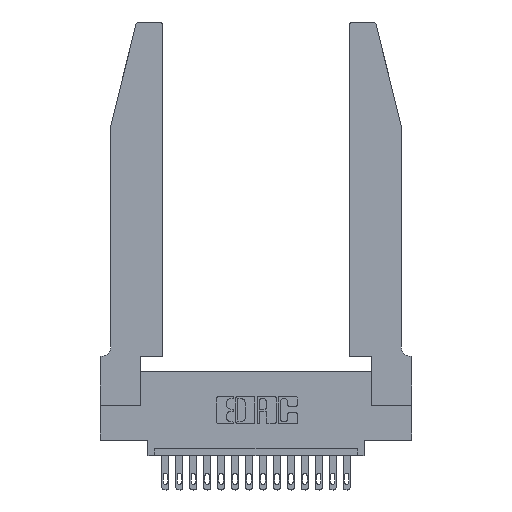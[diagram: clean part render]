
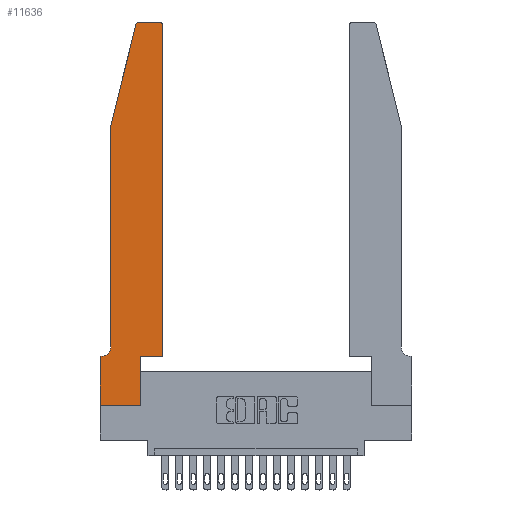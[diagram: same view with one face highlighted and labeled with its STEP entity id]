
A CAD part, top view. The second image highlights one B-rep face of the part: STEP entity #11636.
In plain terms, the highlighted planar face has unit normal (0, 0, 1).
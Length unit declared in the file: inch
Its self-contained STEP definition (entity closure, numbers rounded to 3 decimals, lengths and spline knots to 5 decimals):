
#228 = DIRECTION ( 'NONE',  ( 0., 0., 1. ) ) ;
#827 = LINE ( 'NONE', #8699, #14005 ) ;
#877 = DIRECTION ( 'NONE',  ( 1., 0., 0. ) ) ;
#1120 = VERTEX_POINT ( 'NONE', #11912 ) ;
#1495 = ORIENTED_EDGE ( 'NONE', *, *, #17702, .T. ) ;
#1582 = EDGE_CURVE ( 'NONE', #5676, #4502, #16400, .T. ) ;
#1652 = ORIENTED_EDGE ( 'NONE', *, *, #2172, .T. ) ;
#1903 = VECTOR ( 'NONE', #17147, 39.37008 ) ;
#2052 = VECTOR ( 'NONE', #2347, 39.37008 ) ;
#2172 = EDGE_CURVE ( 'NONE', #15563, #7619, #3936, .T. ) ;
#2191 = EDGE_CURVE ( 'NONE', #11551, #15723, #13420, .T. ) ;
#2324 = VERTEX_POINT ( 'NONE', #4668 ) ;
#2347 = DIRECTION ( 'NONE',  ( -1., 0., 0. ) ) ;
#2508 = EDGE_CURVE ( 'NONE', #11170, #12151, #18224, .T. ) ;
#2566 = VERTEX_POINT ( 'NONE', #10571 ) ;
#2776 = DIRECTION ( 'NONE',  ( 0., 1., 0. ) ) ;
#2810 = VERTEX_POINT ( 'NONE', #17596 ) ;
#2913 = LINE ( 'NONE', #4439, #18145 ) ;
#3308 = LINE ( 'NONE', #15103, #14832 ) ;
#3457 = DIRECTION ( 'NONE',  ( -1., 0., 0. ) ) ;
#3936 = CIRCLE ( 'NONE', #7924, 0.03 ) ;
#4192 = CARTESIAN_POINT ( 'NONE',  ( 0.4505, 0.35, 0.37 ) ) ;
#4439 = CARTESIAN_POINT ( 'NONE',  ( 0.2865, 0.35, 0.37 ) ) ;
#4440 = EDGE_CURVE ( 'NONE', #1120, #2810, #827, .T. ) ;
#4502 = VERTEX_POINT ( 'NONE', #7293 ) ;
#4646 = CARTESIAN_POINT ( 'NONE',  ( 0.4205, 2.75, 0.37 ) ) ;
#4668 = CARTESIAN_POINT ( 'NONE',  ( 0.25487, 2.72718, 0.37 ) ) ;
#4778 = FACE_OUTER_BOUND ( 'NONE', #5576, .T. ) ;
#4799 = EDGE_CURVE ( 'NONE', #2566, #2324, #15820, .T. ) ;
#4938 = EDGE_CURVE ( 'NONE', #2810, #11551, #2913, .T. ) ;
#5576 = EDGE_LOOP ( 'NONE', ( #1495, #14853, #16172, #13009, #5839, #6800, #15413, #8467, #8032, #9935, #11289, #1652 ) ) ;
#5676 = VERTEX_POINT ( 'NONE', #15583 ) ;
#5839 = ORIENTED_EDGE ( 'NONE', *, *, #15623, .T. ) ;
#5838 = CIRCLE ( 'NONE', #8459, 0.07 ) ;
#6117 = CARTESIAN_POINT ( 'NONE',  ( 0.0755, 2., 0.37 ) ) ;
#6229 = CARTESIAN_POINT ( 'NONE',  ( 0.0755, 0.42, 0.37 ) ) ;
#6305 = DIRECTION ( 'NONE',  ( -0.239, -0.971, 0. ) ) ;
#6800 = ORIENTED_EDGE ( 'NONE', *, *, #1582, .T. ) ;
#7256 = VECTOR ( 'NONE', #16569, 39.37008 ) ;
#7293 = CARTESIAN_POINT ( 'NONE',  ( 0., 0.35, 0.37 ) ) ;
#7357 = DIRECTION ( 'NONE',  ( 1., 0., 0. ) ) ;
#7619 = VERTEX_POINT ( 'NONE', #4646 ) ;
#7793 = AXIS2_PLACEMENT_3D ( 'NONE', #13334, #228, #14474 ) ;
#7924 = AXIS2_PLACEMENT_3D ( 'NONE', #17405, #8652, #11590 ) ;
#8032 = ORIENTED_EDGE ( 'NONE', *, *, #4938, .T. ) ;
#8459 = AXIS2_PLACEMENT_3D ( 'NONE', #16717, #12314, #3457 ) ;
#8467 = ORIENTED_EDGE ( 'NONE', *, *, #4440, .T. ) ;
#8590 = LINE ( 'NONE', #13979, #2052 ) ;
#8652 = DIRECTION ( 'NONE',  ( 0., 0., 1. ) ) ;
#8699 = CARTESIAN_POINT ( 'NONE',  ( 0., 0., 0.37 ) ) ;
#9335 = CARTESIAN_POINT ( 'NONE',  ( 0.0755, 0.35, 0.37 ) ) ;
#9536 = AXIS2_PLACEMENT_3D ( 'NONE', #18430, #18363, #877 ) ;
#9935 = ORIENTED_EDGE ( 'NONE', *, *, #2191, .T. ) ;
#10571 = CARTESIAN_POINT ( 'NONE',  ( 0.284, 2.75, 0.37 ) ) ;
#10766 = CARTESIAN_POINT ( 'NONE',  ( 0.4505, 2.72, 0.37 ) ) ;
#11170 = VERTEX_POINT ( 'NONE', #6117 ) ;
#11289 = ORIENTED_EDGE ( 'NONE', *, *, #12926, .T. ) ;
#11365 = VECTOR ( 'NONE', #14392, 39.37008 ) ;
#11551 = VERTEX_POINT ( 'NONE', #17723 ) ;
#11590 = DIRECTION ( 'NONE',  ( 1., 0., 0. ) ) ;
#11636 = ADVANCED_FACE ( 'NONE', ( #4778 ), #19118, .T. ) ;
#11912 = CARTESIAN_POINT ( 'NONE',  ( 0., 0., 0.37 ) ) ;
#12151 = VERTEX_POINT ( 'NONE', #6229 ) ;
#12270 = VECTOR ( 'NONE', #18861, 39.37008 ) ;
#12314 = DIRECTION ( 'NONE',  ( 0., 0., -1. ) ) ;
#12926 = EDGE_CURVE ( 'NONE', #15723, #15563, #15806, .T. ) ;
#13009 = ORIENTED_EDGE ( 'NONE', *, *, #2508, .T. ) ;
#13334 = CARTESIAN_POINT ( 'NONE',  ( 0., 0.35, 0.37 ) ) ;
#13351 = DIRECTION ( 'NONE',  ( 0., 1., 0. ) ) ;
#13420 = LINE ( 'NONE', #4192, #11365 ) ;
#13979 = CARTESIAN_POINT ( 'NONE',  ( 0.2605, 2.75, 0.37 ) ) ;
#14005 = VECTOR ( 'NONE', #7357, 39.37008 ) ;
#14392 = DIRECTION ( 'NONE',  ( 1., 0., 0. ) ) ;
#14474 = DIRECTION ( 'NONE',  ( 1., 0., 0. ) ) ;
#14575 = CARTESIAN_POINT ( 'NONE',  ( 0.0755, 2., 0.37 ) ) ;
#14832 = VECTOR ( 'NONE', #6305, 39.37008 ) ;
#14853 = ORIENTED_EDGE ( 'NONE', *, *, #4799, .T. ) ;
#14986 = EDGE_CURVE ( 'NONE', #2324, #11170, #3308, .T. ) ;
#15011 = EDGE_CURVE ( 'NONE', #4502, #1120, #15294, .T. ) ;
#15103 = CARTESIAN_POINT ( 'NONE',  ( 0.0755, 2., 0.37 ) ) ;
#15294 = LINE ( 'NONE', #17694, #1903 ) ;
#15413 = ORIENTED_EDGE ( 'NONE', *, *, #15011, .T. ) ;
#15505 = CARTESIAN_POINT ( 'NONE',  ( 0.4505, 0.35, 0.37 ) ) ;
#15563 = VERTEX_POINT ( 'NONE', #10766 ) ;
#15583 = CARTESIAN_POINT ( 'NONE',  ( 0.0055, 0.35, 0.37 ) ) ;
#15623 = EDGE_CURVE ( 'NONE', #12151, #5676, #5838, .T. ) ;
#15723 = VERTEX_POINT ( 'NONE', #15505 ) ;
#15806 = LINE ( 'NONE', #17672, #16730 ) ;
#15820 = CIRCLE ( 'NONE', #9536, 0.03 ) ;
#16172 = ORIENTED_EDGE ( 'NONE', *, *, #14986, .T. ) ;
#16400 = LINE ( 'NONE', #9335, #7256 ) ;
#16569 = DIRECTION ( 'NONE',  ( -1., 0., 0. ) ) ;
#16717 = CARTESIAN_POINT ( 'NONE',  ( 0.0055, 0.42, 0.37 ) ) ;
#16730 = VECTOR ( 'NONE', #2776, 39.37008 ) ;
#17147 = DIRECTION ( 'NONE',  ( 0., -1., 0. ) ) ;
#17405 = CARTESIAN_POINT ( 'NONE',  ( 0.4205, 2.72, 0.37 ) ) ;
#17596 = CARTESIAN_POINT ( 'NONE',  ( 0.2865, 0., 0.37 ) ) ;
#17672 = CARTESIAN_POINT ( 'NONE',  ( 0.4505, 0.35, 0.37 ) ) ;
#17694 = CARTESIAN_POINT ( 'NONE',  ( 0., 0., 0.37 ) ) ;
#17702 = EDGE_CURVE ( 'NONE', #7619, #2566, #8590, .T. ) ;
#17723 = CARTESIAN_POINT ( 'NONE',  ( 0.2865, 0.35, 0.37 ) ) ;
#18145 = VECTOR ( 'NONE', #13351, 39.37008 ) ;
#18224 = LINE ( 'NONE', #14575, #12270 ) ;
#18363 = DIRECTION ( 'NONE',  ( 0., 0., 1. ) ) ;
#18430 = CARTESIAN_POINT ( 'NONE',  ( 0.284, 2.72, 0.37 ) ) ;
#18861 = DIRECTION ( 'NONE',  ( 0., -1., 0. ) ) ;
#19118 = PLANE ( 'NONE',  #7793 ) ;
